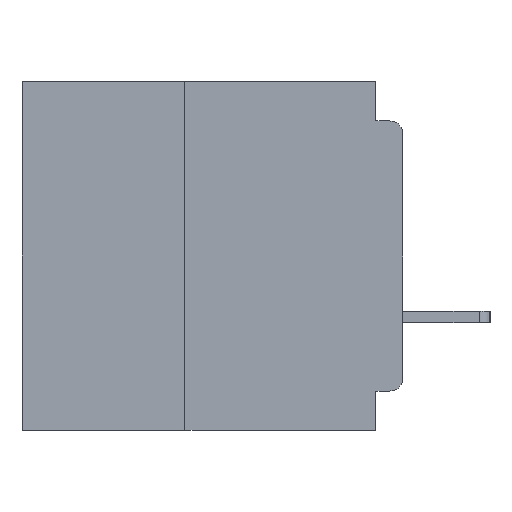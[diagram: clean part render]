
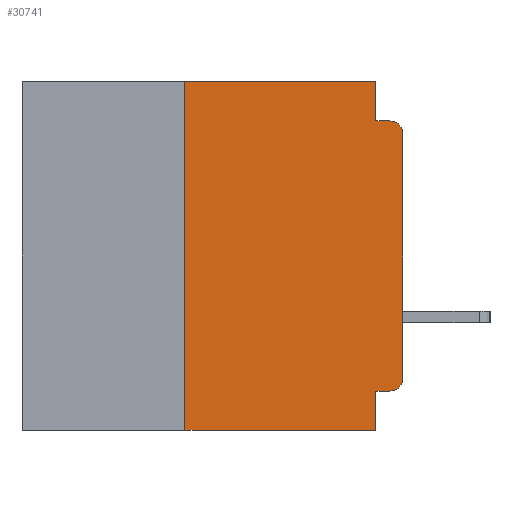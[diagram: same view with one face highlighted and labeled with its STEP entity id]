
A CAD part, left-side view. The second image highlights one B-rep face of the part: STEP entity #30741.
In plain terms, the highlighted planar face has unit normal (-1, 0, 0).
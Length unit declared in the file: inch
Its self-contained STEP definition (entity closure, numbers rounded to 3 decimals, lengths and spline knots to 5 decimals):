
#179 = DIRECTION ( 'NONE',  ( 0., 1., 0. ) ) ;
#531 = ORIENTED_EDGE ( 'NONE', *, *, #17348, .T. ) ;
#790 = EDGE_CURVE ( 'NONE', #35539, #32871, #7269, .T. ) ;
#1065 = CARTESIAN_POINT ( 'NONE',  ( 0., 0.031, -0.4 ) ) ;
#1331 = VERTEX_POINT ( 'NONE', #19486 ) ;
#1596 = VERTEX_POINT ( 'NONE', #2534 ) ;
#2534 = CARTESIAN_POINT ( 'NONE',  ( 0., 0.031, 0. ) ) ;
#2736 = CARTESIAN_POINT ( 'NONE',  ( 0., 0.031, -0.045 ) ) ;
#2992 = CARTESIAN_POINT ( 'NONE',  ( 0., 0.015, -0.045 ) ) ;
#3535 = VECTOR ( 'NONE', #179, 39.37008 ) ;
#3654 = DIRECTION ( 'NONE',  ( 0., 0., 1. ) ) ;
#3699 = CARTESIAN_POINT ( 'NONE',  ( 0., 0., -0.355 ) ) ;
#3813 = VECTOR ( 'NONE', #17962, 39.37008 ) ;
#4100 = CARTESIAN_POINT ( 'NONE',  ( 0., 0.25, -0.4 ) ) ;
#4288 = DIRECTION ( 'NONE',  ( 0., 0., -1. ) ) ;
#5271 = EDGE_LOOP ( 'NONE', ( #25901, #19023, #13106, #24349, #12589, #7750, #37100, #11469, #21652, #531 ) ) ;
#5300 = DIRECTION ( 'NONE',  ( -1., 0., 0. ) ) ;
#6865 = DIRECTION ( 'NONE',  ( 0., -1., 0. ) ) ;
#7269 = LINE ( 'NONE', #4100, #42482 ) ;
#7429 = LINE ( 'NONE', #41962, #35712 ) ;
#7750 = ORIENTED_EDGE ( 'NONE', *, *, #790, .F. ) ;
#8292 = CARTESIAN_POINT ( 'NONE',  ( 0., 0.015, -0.06 ) ) ;
#9170 = VECTOR ( 'NONE', #17608, 39.37008 ) ;
#10175 = CARTESIAN_POINT ( 'NONE',  ( 0., 0., -0.045 ) ) ;
#11035 = CARTESIAN_POINT ( 'NONE',  ( 0., 0.437, 0. ) ) ;
#11469 = ORIENTED_EDGE ( 'NONE', *, *, #12881, .F. ) ;
#11474 = PLANE ( 'NONE',  #29872 ) ;
#11759 = DIRECTION ( 'NONE',  ( 0., 0., -1. ) ) ;
#12007 = CARTESIAN_POINT ( 'NONE',  ( 0., 0., -0.34 ) ) ;
#12589 = ORIENTED_EDGE ( 'NONE', *, *, #28016, .F. ) ;
#12881 = EDGE_CURVE ( 'NONE', #1331, #13198, #24628, .T. ) ;
#13106 = ORIENTED_EDGE ( 'NONE', *, *, #34330, .F. ) ;
#13198 = VERTEX_POINT ( 'NONE', #33411 ) ;
#15249 = LINE ( 'NONE', #10175, #41316 ) ;
#15651 = VERTEX_POINT ( 'NONE', #2992 ) ;
#16226 = CARTESIAN_POINT ( 'NONE',  ( 0., 0.25, -0.4 ) ) ;
#17075 = CARTESIAN_POINT ( 'NONE',  ( 0., 0., -0.06 ) ) ;
#17348 = EDGE_CURVE ( 'NONE', #24944, #40952, #27040, .T. ) ;
#17608 = DIRECTION ( 'NONE',  ( 0., 0., 1. ) ) ;
#17962 = DIRECTION ( 'NONE',  ( 0., -1., 0. ) ) ;
#18387 = DIRECTION ( 'NONE',  ( 0., 0., -1. ) ) ;
#19023 = ORIENTED_EDGE ( 'NONE', *, *, #19176, .T. ) ;
#19176 = EDGE_CURVE ( 'NONE', #40240, #15651, #36969, .T. ) ;
#19486 = CARTESIAN_POINT ( 'NONE',  ( 0., 0.031, -0.355 ) ) ;
#20356 = CARTESIAN_POINT ( 'NONE',  ( 0., 0.437, -0.4 ) ) ;
#21652 = ORIENTED_EDGE ( 'NONE', *, *, #25277, .F. ) ;
#21824 = EDGE_CURVE ( 'NONE', #1596, #23882, #7429, .T. ) ;
#22876 = EDGE_CURVE ( 'NONE', #35539, #13198, #33158, .T. ) ;
#23882 = VERTEX_POINT ( 'NONE', #2736 ) ;
#24349 = ORIENTED_EDGE ( 'NONE', *, *, #21824, .F. ) ;
#24443 = CARTESIAN_POINT ( 'NONE',  ( 0., 0., 0. ) ) ;
#24628 = LINE ( 'NONE', #1065, #33622 ) ;
#24944 = VERTEX_POINT ( 'NONE', #32604 ) ;
#25209 = VECTOR ( 'NONE', #44084, 39.37008 ) ;
#25277 = EDGE_CURVE ( 'NONE', #24944, #1331, #31931, .T. ) ;
#25836 = CARTESIAN_POINT ( 'NONE',  ( 0., 0.015, -0.34 ) ) ;
#25901 = ORIENTED_EDGE ( 'NONE', *, *, #35186, .T. ) ;
#27040 = CIRCLE ( 'NONE', #37740, 0.015 ) ;
#28016 = EDGE_CURVE ( 'NONE', #32871, #1596, #39148, .T. ) ;
#29254 = DIRECTION ( 'NONE',  ( 0., 0., -1. ) ) ;
#29872 = AXIS2_PLACEMENT_3D ( 'NONE', #35291, #38742, #18387 ) ;
#30741 = ADVANCED_FACE ( 'NONE', ( #37309 ), #11474, .F. ) ;
#31931 = LINE ( 'NONE', #3699, #3535 ) ;
#32155 = DIRECTION ( 'NONE',  ( -1., 0., 0. ) ) ;
#32604 = CARTESIAN_POINT ( 'NONE',  ( 0., 0.015, -0.355 ) ) ;
#32871 = VERTEX_POINT ( 'NONE', #35911 ) ;
#33158 = LINE ( 'NONE', #20356, #25209 ) ;
#33411 = CARTESIAN_POINT ( 'NONE',  ( 0., 0.031, -0.4 ) ) ;
#33622 = VECTOR ( 'NONE', #4288, 39.37008 ) ;
#34330 = EDGE_CURVE ( 'NONE', #23882, #15651, #15249, .T. ) ;
#35186 = EDGE_CURVE ( 'NONE', #40952, #40240, #36370, .T. ) ;
#35291 = CARTESIAN_POINT ( 'NONE',  ( 0., 0.437, 0. ) ) ;
#35539 = VERTEX_POINT ( 'NONE', #16226 ) ;
#35712 = VECTOR ( 'NONE', #38552, 39.37008 ) ;
#35911 = CARTESIAN_POINT ( 'NONE',  ( 0., 0.25, 0. ) ) ;
#36370 = LINE ( 'NONE', #24443, #9170 ) ;
#36969 = CIRCLE ( 'NONE', #43197, 0.015 ) ;
#37100 = ORIENTED_EDGE ( 'NONE', *, *, #22876, .T. ) ;
#37309 = FACE_OUTER_BOUND ( 'NONE', #5271, .T. ) ;
#37740 = AXIS2_PLACEMENT_3D ( 'NONE', #25836, #5300, #29254 ) ;
#38552 = DIRECTION ( 'NONE',  ( 0., 0., -1. ) ) ;
#38742 = DIRECTION ( 'NONE',  ( 1., 0., 0. ) ) ;
#39148 = LINE ( 'NONE', #11035, #3813 ) ;
#40240 = VERTEX_POINT ( 'NONE', #17075 ) ;
#40952 = VERTEX_POINT ( 'NONE', #12007 ) ;
#41316 = VECTOR ( 'NONE', #6865, 39.37008 ) ;
#41962 = CARTESIAN_POINT ( 'NONE',  ( 0., 0.031, 0. ) ) ;
#42482 = VECTOR ( 'NONE', #3654, 39.37008 ) ;
#43197 = AXIS2_PLACEMENT_3D ( 'NONE', #8292, #32155, #11759 ) ;
#44084 = DIRECTION ( 'NONE',  ( 0., -1., 0. ) ) ;
